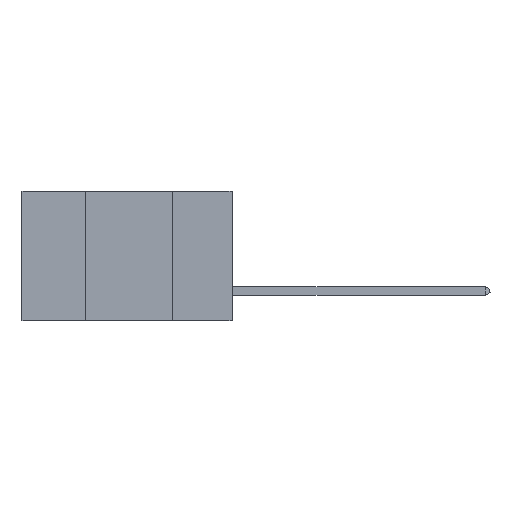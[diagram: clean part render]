
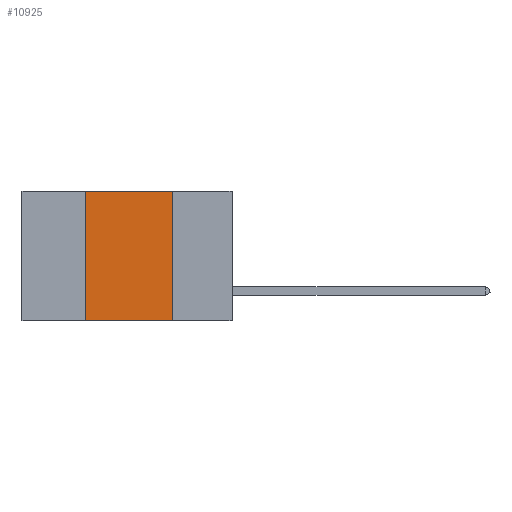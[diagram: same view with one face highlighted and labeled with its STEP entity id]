
A CAD part, left-side view. The second image highlights one B-rep face of the part: STEP entity #10925.
In plain terms, the highlighted planar face has unit normal (-1, 0, 0).
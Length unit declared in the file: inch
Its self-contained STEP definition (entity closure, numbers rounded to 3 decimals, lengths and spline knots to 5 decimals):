
#506 = DIRECTION ( 'NONE',  ( 0., 0., -1. ) ) ;
#583 = LINE ( 'NONE', #2995, #9566 ) ;
#1400 = DIRECTION ( 'NONE',  ( 0., 0., -1. ) ) ;
#1525 = ORIENTED_EDGE ( 'NONE', *, *, #6577, .F. ) ;
#1888 = AXIS2_PLACEMENT_3D ( 'NONE', #4004, #5736, #506 ) ;
#2184 = CARTESIAN_POINT ( 'NONE',  ( 0., 0.6, -0.37 ) ) ;
#2545 = FACE_OUTER_BOUND ( 'NONE', #11254, .T. ) ;
#2717 = LINE ( 'NONE', #2184, #8972 ) ;
#2995 = CARTESIAN_POINT ( 'NONE',  ( 0., 0.6, 0. ) ) ;
#3413 = VERTEX_POINT ( 'NONE', #11024 ) ;
#3610 = ORIENTED_EDGE ( 'NONE', *, *, #5302, .F. ) ;
#3681 = ORIENTED_EDGE ( 'NONE', *, *, #7216, .F. ) ;
#4004 = CARTESIAN_POINT ( 'NONE',  ( 0., 0.6, 0. ) ) ;
#4036 = CARTESIAN_POINT ( 'NONE',  ( 0., 0.17, 0. ) ) ;
#4581 = VERTEX_POINT ( 'NONE', #6032 ) ;
#4906 = VECTOR ( 'NONE', #1400, 39.37008 ) ;
#5190 = LINE ( 'NONE', #9991, #6554 ) ;
#5302 = EDGE_CURVE ( 'NONE', #4581, #10130, #583, .T. ) ;
#5736 = DIRECTION ( 'NONE',  ( 1., 0., 0. ) ) ;
#6032 = CARTESIAN_POINT ( 'NONE',  ( 0., 0.42, 0. ) ) ;
#6554 = VECTOR ( 'NONE', #9049, 39.37008 ) ;
#6577 = EDGE_CURVE ( 'NONE', #8031, #4581, #5190, .T. ) ;
#6883 = CARTESIAN_POINT ( 'NONE',  ( 0., 0.42, -0.37 ) ) ;
#7116 = EDGE_CURVE ( 'NONE', #8031, #3413, #2717, .T. ) ;
#7216 = EDGE_CURVE ( 'NONE', #10130, #3413, #11168, .T. ) ;
#7359 = CARTESIAN_POINT ( 'NONE',  ( 0., 0.17, 0. ) ) ;
#8031 = VERTEX_POINT ( 'NONE', #6883 ) ;
#8972 = VECTOR ( 'NONE', #10914, 39.37008 ) ;
#9049 = DIRECTION ( 'NONE',  ( 0., 0., 1. ) ) ;
#9566 = VECTOR ( 'NONE', #9976, 39.37008 ) ;
#9976 = DIRECTION ( 'NONE',  ( 0., -1., 0. ) ) ;
#9991 = CARTESIAN_POINT ( 'NONE',  ( 0., 0.42, 0. ) ) ;
#10011 = PLANE ( 'NONE',  #1888 ) ;
#10130 = VERTEX_POINT ( 'NONE', #7359 ) ;
#10319 = ORIENTED_EDGE ( 'NONE', *, *, #7116, .T. ) ;
#10914 = DIRECTION ( 'NONE',  ( 0., -1., 0. ) ) ;
#10925 = ADVANCED_FACE ( 'NONE', ( #2545 ), #10011, .F. ) ;
#11024 = CARTESIAN_POINT ( 'NONE',  ( 0., 0.17, -0.37 ) ) ;
#11168 = LINE ( 'NONE', #4036, #4906 ) ;
#11254 = EDGE_LOOP ( 'NONE', ( #3681, #3610, #1525, #10319 ) ) ;
